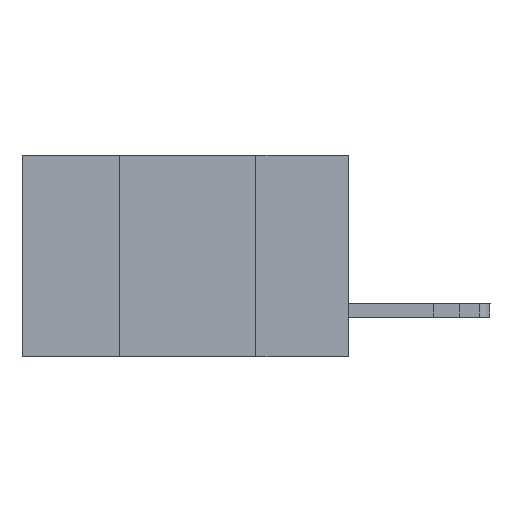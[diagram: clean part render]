
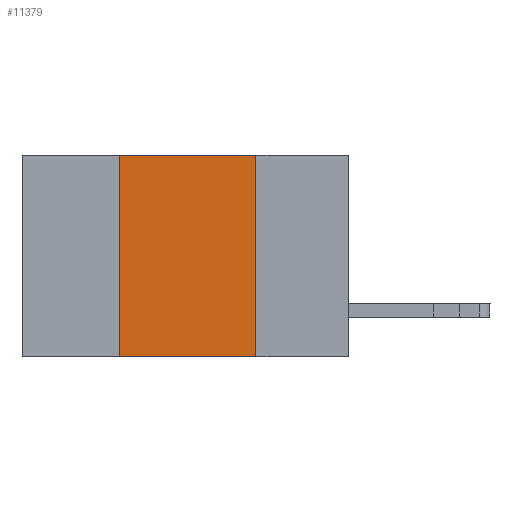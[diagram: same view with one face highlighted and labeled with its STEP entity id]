
A CAD part, left-side view. The second image highlights one B-rep face of the part: STEP entity #11379.
In plain terms, the highlighted planar face has unit normal (-1, 0, 0).
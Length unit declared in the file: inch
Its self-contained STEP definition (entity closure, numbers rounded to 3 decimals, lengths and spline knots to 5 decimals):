
#409 = CARTESIAN_POINT ( 'NONE',  ( 0., 0.42, 0. ) ) ;
#1260 = LINE ( 'NONE', #409, #10929 ) ;
#1430 = PLANE ( 'NONE',  #12834 ) ;
#1538 = EDGE_LOOP ( 'NONE', ( #3985, #9771, #1953, #7163 ) ) ;
#1953 = ORIENTED_EDGE ( 'NONE', *, *, #2599, .F. ) ;
#2599 = EDGE_CURVE ( 'NONE', #8304, #11756, #1260, .T. ) ;
#2806 = CARTESIAN_POINT ( 'NONE',  ( 0., 0.6, 0. ) ) ;
#3178 = DIRECTION ( 'NONE',  ( 0., 0., -1. ) ) ;
#3217 = DIRECTION ( 'NONE',  ( 0., 0., 1. ) ) ;
#3738 = EDGE_CURVE ( 'NONE', #11756, #4255, #10379, .T. ) ;
#3849 = DIRECTION ( 'NONE',  ( 1., 0., 0. ) ) ;
#3985 = ORIENTED_EDGE ( 'NONE', *, *, #6036, .F. ) ;
#4255 = VERTEX_POINT ( 'NONE', #6065 ) ;
#4698 = FACE_OUTER_BOUND ( 'NONE', #1538, .T. ) ;
#5517 = CARTESIAN_POINT ( 'NONE',  ( 0., 0.6, 0. ) ) ;
#6036 = EDGE_CURVE ( 'NONE', #4255, #12453, #12207, .T. ) ;
#6065 = CARTESIAN_POINT ( 'NONE',  ( 0., 0.17, 0. ) ) ;
#6361 = CARTESIAN_POINT ( 'NONE',  ( 0., 0.17, 0. ) ) ;
#6730 = CARTESIAN_POINT ( 'NONE',  ( 0., 0.42, 0. ) ) ;
#7163 = ORIENTED_EDGE ( 'NONE', *, *, #8861, .T. ) ;
#8211 = CARTESIAN_POINT ( 'NONE',  ( 0., 0.42, -0.37 ) ) ;
#8304 = VERTEX_POINT ( 'NONE', #8211 ) ;
#8577 = LINE ( 'NONE', #9682, #9524 ) ;
#8847 = VECTOR ( 'NONE', #10642, 39.37008 ) ;
#8861 = EDGE_CURVE ( 'NONE', #8304, #12453, #8577, .T. ) ;
#9524 = VECTOR ( 'NONE', #12609, 39.37008 ) ;
#9682 = CARTESIAN_POINT ( 'NONE',  ( 0., 0.6, -0.37 ) ) ;
#9771 = ORIENTED_EDGE ( 'NONE', *, *, #3738, .F. ) ;
#10197 = CARTESIAN_POINT ( 'NONE',  ( 0., 0.17, -0.37 ) ) ;
#10379 = LINE ( 'NONE', #5517, #8847 ) ;
#10642 = DIRECTION ( 'NONE',  ( 0., -1., 0. ) ) ;
#10682 = VECTOR ( 'NONE', #12327, 39.37008 ) ;
#10929 = VECTOR ( 'NONE', #3217, 39.37008 ) ;
#11379 = ADVANCED_FACE ( 'NONE', ( #4698 ), #1430, .F. ) ;
#11756 = VERTEX_POINT ( 'NONE', #6730 ) ;
#12207 = LINE ( 'NONE', #6361, #10682 ) ;
#12327 = DIRECTION ( 'NONE',  ( 0., 0., -1. ) ) ;
#12453 = VERTEX_POINT ( 'NONE', #10197 ) ;
#12609 = DIRECTION ( 'NONE',  ( 0., -1., 0. ) ) ;
#12834 = AXIS2_PLACEMENT_3D ( 'NONE', #2806, #3849, #3178 ) ;
